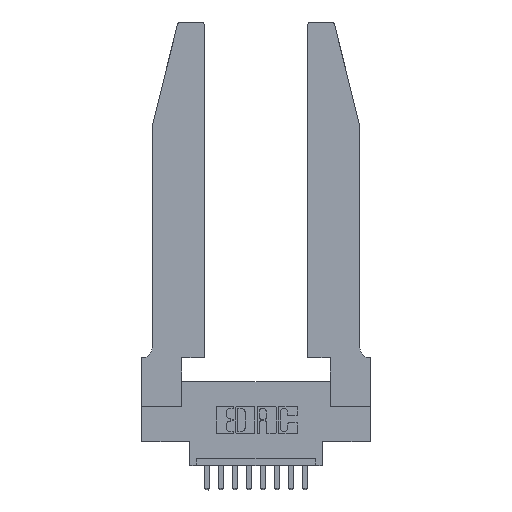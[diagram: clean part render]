
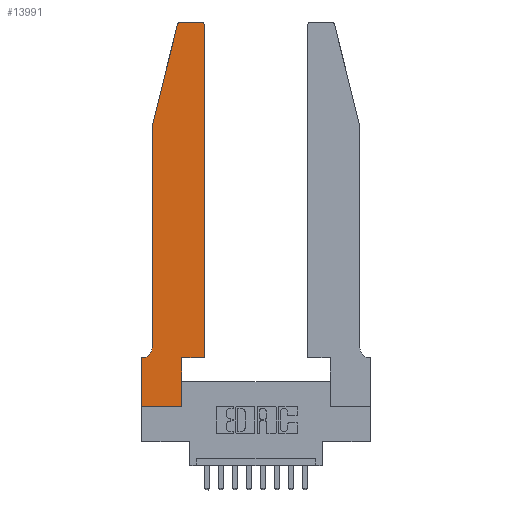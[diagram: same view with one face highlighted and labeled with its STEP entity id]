
A CAD part, top view. The second image highlights one B-rep face of the part: STEP entity #13991.
In plain terms, the highlighted planar face has unit normal (0, 0, 1).
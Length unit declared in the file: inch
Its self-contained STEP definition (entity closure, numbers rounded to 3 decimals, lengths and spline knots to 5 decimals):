
#105 = EDGE_LOOP ( 'NONE', ( #15015, #8228, #3105, #9794, #9032, #15577, #5456, #2617, #12726, #14349, #14798, #13883 ) ) ;
#733 = DIRECTION ( 'NONE',  ( 0., 0., 1. ) ) ;
#788 = VERTEX_POINT ( 'NONE', #3225 ) ;
#1093 = CARTESIAN_POINT ( 'NONE',  ( 0.0755, 2., 0.37 ) ) ;
#1422 = CARTESIAN_POINT ( 'NONE',  ( 0.4205, 2.72, 0.37 ) ) ;
#1510 = CARTESIAN_POINT ( 'NONE',  ( 0.284, 2.75, 0.37 ) ) ;
#1553 = LINE ( 'NONE', #4555, #6608 ) ;
#1628 = VERTEX_POINT ( 'NONE', #1784 ) ;
#1677 = VECTOR ( 'NONE', #3610, 39.37008 ) ;
#1689 = CARTESIAN_POINT ( 'NONE',  ( 0.0755, 2., 0.37 ) ) ;
#1784 = CARTESIAN_POINT ( 'NONE',  ( 0.2865, 0.35, 0.37 ) ) ;
#1939 = DIRECTION ( 'NONE',  ( 0., 1., 0. ) ) ;
#2299 = VERTEX_POINT ( 'NONE', #1510 ) ;
#2325 = CARTESIAN_POINT ( 'NONE',  ( 0., 0.35, 0.37 ) ) ;
#2500 = AXIS2_PLACEMENT_3D ( 'NONE', #5582, #8239, #14195 ) ;
#2538 = AXIS2_PLACEMENT_3D ( 'NONE', #13369, #11009, #12143 ) ;
#2617 = ORIENTED_EDGE ( 'NONE', *, *, #15338, .T. ) ;
#2800 = EDGE_CURVE ( 'NONE', #3354, #5508, #6950, .T. ) ;
#2860 = LINE ( 'NONE', #12665, #12917 ) ;
#2907 = CARTESIAN_POINT ( 'NONE',  ( 0.0055, 0.35, 0.37 ) ) ;
#3105 = ORIENTED_EDGE ( 'NONE', *, *, #13896, .T. ) ;
#3225 = CARTESIAN_POINT ( 'NONE',  ( 0.25487, 2.72718, 0.37 ) ) ;
#3354 = VERTEX_POINT ( 'NONE', #8548 ) ;
#3610 = DIRECTION ( 'NONE',  ( -1., 0., 0. ) ) ;
#3760 = VECTOR ( 'NONE', #7899, 39.37008 ) ;
#3771 = EDGE_CURVE ( 'NONE', #15386, #12578, #10342, .T. ) ;
#3859 = DIRECTION ( 'NONE',  ( 0., 0., 1. ) ) ;
#3895 = VECTOR ( 'NONE', #14776, 39.37008 ) ;
#4477 = EDGE_CURVE ( 'NONE', #10871, #15386, #12802, .T. ) ;
#4555 = CARTESIAN_POINT ( 'NONE',  ( 0., 0., 0.37 ) ) ;
#4564 = CARTESIAN_POINT ( 'NONE',  ( 0.0755, 0.42, 0.37 ) ) ;
#4800 = CARTESIAN_POINT ( 'NONE',  ( 0.2605, 2.75, 0.37 ) ) ;
#5133 = VERTEX_POINT ( 'NONE', #8885 ) ;
#5456 = ORIENTED_EDGE ( 'NONE', *, *, #14599, .T. ) ;
#5508 = VERTEX_POINT ( 'NONE', #12211 ) ;
#5568 = EDGE_CURVE ( 'NONE', #11980, #2299, #7063, .T. ) ;
#5582 = CARTESIAN_POINT ( 'NONE',  ( 0., 0.35, 0.37 ) ) ;
#5585 = CIRCLE ( 'NONE', #8734, 0.03 ) ;
#5657 = EDGE_CURVE ( 'NONE', #9753, #1628, #6861, .T. ) ;
#6027 = AXIS2_PLACEMENT_3D ( 'NONE', #1422, #3859, #6441 ) ;
#6238 = EDGE_CURVE ( 'NONE', #7551, #10871, #8618, .T. ) ;
#6268 = EDGE_CURVE ( 'NONE', #5508, #11980, #15597, .T. ) ;
#6441 = DIRECTION ( 'NONE',  ( 1., 0., 0. ) ) ;
#6608 = VECTOR ( 'NONE', #8215, 39.37008 ) ;
#6861 = LINE ( 'NONE', #12717, #9915 ) ;
#6950 = LINE ( 'NONE', #15125, #3760 ) ;
#7063 = LINE ( 'NONE', #4800, #14112 ) ;
#7519 = DIRECTION ( 'NONE',  ( 1., 0., 0. ) ) ;
#7551 = VERTEX_POINT ( 'NONE', #1093 ) ;
#7556 = CARTESIAN_POINT ( 'NONE',  ( 0.4505, 0.35, 0.37 ) ) ;
#7607 = DIRECTION ( 'NONE',  ( 1., 0., 0. ) ) ;
#7899 = DIRECTION ( 'NONE',  ( 0., 1., 0. ) ) ;
#8215 = DIRECTION ( 'NONE',  ( 0., -1., 0. ) ) ;
#8228 = ORIENTED_EDGE ( 'NONE', *, *, #11698, .T. ) ;
#8239 = DIRECTION ( 'NONE',  ( 0., 0., 1. ) ) ;
#8548 = CARTESIAN_POINT ( 'NONE',  ( 0.4505, 0.35, 0.37 ) ) ;
#8618 = LINE ( 'NONE', #1689, #3895 ) ;
#8664 = LINE ( 'NONE', #7556, #9617 ) ;
#8734 = AXIS2_PLACEMENT_3D ( 'NONE', #14202, #733, #11553 ) ;
#8885 = CARTESIAN_POINT ( 'NONE',  ( 0., 0., 0.37 ) ) ;
#9032 = ORIENTED_EDGE ( 'NONE', *, *, #4477, .T. ) ;
#9617 = VECTOR ( 'NONE', #7607, 39.37008 ) ;
#9753 = VERTEX_POINT ( 'NONE', #10600 ) ;
#9794 = ORIENTED_EDGE ( 'NONE', *, *, #6238, .T. ) ;
#9915 = VECTOR ( 'NONE', #1939, 39.37008 ) ;
#10342 = LINE ( 'NONE', #14667, #1677 ) ;
#10522 = PLANE ( 'NONE',  #2500 ) ;
#10573 = EDGE_CURVE ( 'NONE', #1628, #3354, #8664, .T. ) ;
#10600 = CARTESIAN_POINT ( 'NONE',  ( 0.2865, 0., 0.37 ) ) ;
#10871 = VERTEX_POINT ( 'NONE', #4564 ) ;
#11009 = DIRECTION ( 'NONE',  ( 0., 0., -1. ) ) ;
#11553 = DIRECTION ( 'NONE',  ( 1., 0., 0. ) ) ;
#11593 = DIRECTION ( 'NONE',  ( -0.239, -0.971, 0. ) ) ;
#11698 = EDGE_CURVE ( 'NONE', #2299, #788, #5585, .T. ) ;
#11859 = CARTESIAN_POINT ( 'NONE',  ( 0.4205, 2.75, 0.37 ) ) ;
#11980 = VERTEX_POINT ( 'NONE', #11859 ) ;
#12143 = DIRECTION ( 'NONE',  ( -1., 0., 0. ) ) ;
#12211 = CARTESIAN_POINT ( 'NONE',  ( 0.4505, 2.72, 0.37 ) ) ;
#12578 = VERTEX_POINT ( 'NONE', #2325 ) ;
#12665 = CARTESIAN_POINT ( 'NONE',  ( 0.0755, 2., 0.37 ) ) ;
#12717 = CARTESIAN_POINT ( 'NONE',  ( 0.2865, 0.35, 0.37 ) ) ;
#12726 = ORIENTED_EDGE ( 'NONE', *, *, #5657, .T. ) ;
#12802 = CIRCLE ( 'NONE', #2538, 0.07 ) ;
#12917 = VECTOR ( 'NONE', #11593, 39.37008 ) ;
#13052 = VECTOR ( 'NONE', #7519, 39.37008 ) ;
#13369 = CARTESIAN_POINT ( 'NONE',  ( 0.0055, 0.42, 0.37 ) ) ;
#13543 = CARTESIAN_POINT ( 'NONE',  ( 0., 0., 0.37 ) ) ;
#13826 = LINE ( 'NONE', #13543, #13052 ) ;
#13883 = ORIENTED_EDGE ( 'NONE', *, *, #6268, .T. ) ;
#13896 = EDGE_CURVE ( 'NONE', #788, #7551, #2860, .T. ) ;
#13991 = ADVANCED_FACE ( 'NONE', ( #14612 ), #10522, .T. ) ;
#14112 = VECTOR ( 'NONE', #14626, 39.37008 ) ;
#14195 = DIRECTION ( 'NONE',  ( 1., 0., 0. ) ) ;
#14202 = CARTESIAN_POINT ( 'NONE',  ( 0.284, 2.72, 0.37 ) ) ;
#14349 = ORIENTED_EDGE ( 'NONE', *, *, #10573, .T. ) ;
#14599 = EDGE_CURVE ( 'NONE', #12578, #5133, #1553, .T. ) ;
#14612 = FACE_OUTER_BOUND ( 'NONE', #105, .T. ) ;
#14626 = DIRECTION ( 'NONE',  ( -1., 0., 0. ) ) ;
#14667 = CARTESIAN_POINT ( 'NONE',  ( 0.0755, 0.35, 0.37 ) ) ;
#14776 = DIRECTION ( 'NONE',  ( 0., -1., 0. ) ) ;
#14798 = ORIENTED_EDGE ( 'NONE', *, *, #2800, .T. ) ;
#15015 = ORIENTED_EDGE ( 'NONE', *, *, #5568, .T. ) ;
#15125 = CARTESIAN_POINT ( 'NONE',  ( 0.4505, 0.35, 0.37 ) ) ;
#15338 = EDGE_CURVE ( 'NONE', #5133, #9753, #13826, .T. ) ;
#15386 = VERTEX_POINT ( 'NONE', #2907 ) ;
#15577 = ORIENTED_EDGE ( 'NONE', *, *, #3771, .T. ) ;
#15597 = CIRCLE ( 'NONE', #6027, 0.03 ) ;
